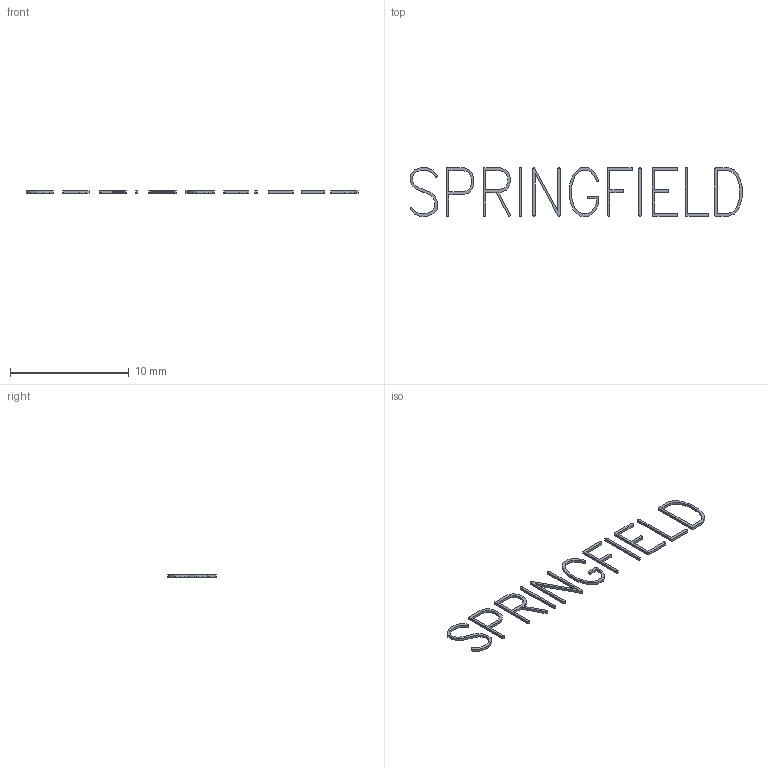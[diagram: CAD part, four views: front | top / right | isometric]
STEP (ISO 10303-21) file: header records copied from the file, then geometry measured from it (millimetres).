
FILE_DESCRIPTION (( 'STEP AP214' ), '1' );
FILE_NAME ('ENGRAVING FILL - SPRINGFIELD.STEP', '2013-06-19T14:04:12', ( 'Asher' ), ( '' ), 'SwSTEP 2.0', 'SolidWorks 2013', '' );
FILE_SCHEMA (( 'AUTOMOTIVE_DESIGN' ));
Length unit declared in the file: millimetre
Products named in the file (1): ENGRAVING FILL - SPRINGFIELD
Bounding box: 27.99 x 4.11 x 0.2 mm (x, y, z)
Volume: 4 mm3; surface area: 77 mm2
Topology: 11 solids, 11 shells, 277 faces, 765 edges, 510 vertices
Faces by surface type: plane 201, bspline 76
Entity records: 10055 total; most frequent: CARTESIAN_POINT 3365, ORIENTED_EDGE 1530, DIRECTION 1017, EDGE_CURVE 765, VECTOR 613, LINE 613, VERTEX_POINT 510, EDGE_LOOP 283
